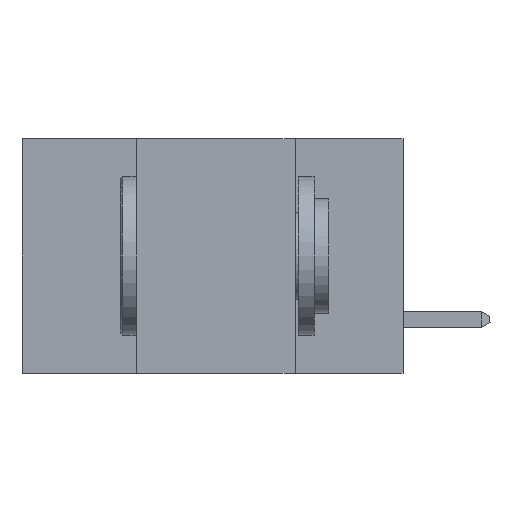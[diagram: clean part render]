
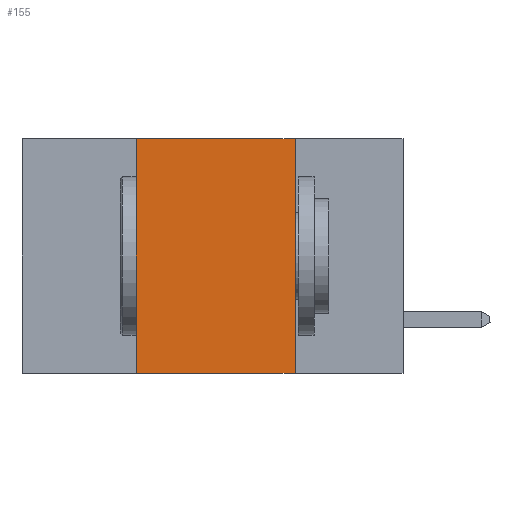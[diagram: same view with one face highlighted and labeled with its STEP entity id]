
A CAD part, left-side view. The second image highlights one B-rep face of the part: STEP entity #155.
In plain terms, the highlighted planar face has unit normal (-1, 0, 0).
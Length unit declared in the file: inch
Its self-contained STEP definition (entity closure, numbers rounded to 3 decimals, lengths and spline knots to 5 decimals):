
#155 = ADVANCED_FACE ( 'NONE', ( #1141 ), #7700, .F. ) ;
#547 = VERTEX_POINT ( 'NONE', #8016 ) ;
#861 = CARTESIAN_POINT ( 'NONE',  ( 0., 0.42, 0. ) ) ;
#939 = DIRECTION ( 'NONE',  ( 0., 0., -1. ) ) ;
#1141 = FACE_OUTER_BOUND ( 'NONE', #3780, .T. ) ;
#1144 = ORIENTED_EDGE ( 'NONE', *, *, #3062, .F. ) ;
#1249 = AXIS2_PLACEMENT_3D ( 'NONE', #10570, #8651, #9579 ) ;
#1253 = DIRECTION ( 'NONE',  ( 0., 0., 1. ) ) ;
#1817 = VERTEX_POINT ( 'NONE', #10960 ) ;
#2206 = EDGE_CURVE ( 'NONE', #1817, #547, #7486, .T. ) ;
#2218 = VECTOR ( 'NONE', #1253, 39.37008 ) ;
#2542 = VECTOR ( 'NONE', #939, 39.37008 ) ;
#3062 = EDGE_CURVE ( 'NONE', #9402, #5827, #3836, .T. ) ;
#3548 = EDGE_CURVE ( 'NONE', #5827, #1817, #9509, .T. ) ;
#3780 = EDGE_LOOP ( 'NONE', ( #6567, #8626, #1144, #9054 ) ) ;
#3836 = LINE ( 'NONE', #10677, #2218 ) ;
#4989 = EDGE_CURVE ( 'NONE', #9402, #547, #8886, .T. ) ;
#5162 = CARTESIAN_POINT ( 'NONE',  ( 0., 0.6, 0. ) ) ;
#5827 = VERTEX_POINT ( 'NONE', #861 ) ;
#5894 = DIRECTION ( 'NONE',  ( 0., -1., 0. ) ) ;
#6567 = ORIENTED_EDGE ( 'NONE', *, *, #2206, .F. ) ;
#7486 = LINE ( 'NONE', #8471, #2542 ) ;
#7700 = PLANE ( 'NONE',  #1249 ) ;
#8016 = CARTESIAN_POINT ( 'NONE',  ( 0., 0.17, -0.37 ) ) ;
#8092 = DIRECTION ( 'NONE',  ( 0., -1., 0. ) ) ;
#8471 = CARTESIAN_POINT ( 'NONE',  ( 0., 0.17, 0. ) ) ;
#8602 = VECTOR ( 'NONE', #5894, 39.37008 ) ;
#8626 = ORIENTED_EDGE ( 'NONE', *, *, #3548, .F. ) ;
#8651 = DIRECTION ( 'NONE',  ( 1., 0., 0. ) ) ;
#8886 = LINE ( 'NONE', #10516, #8602 ) ;
#9054 = ORIENTED_EDGE ( 'NONE', *, *, #4989, .T. ) ;
#9217 = VECTOR ( 'NONE', #8092, 39.37008 ) ;
#9402 = VERTEX_POINT ( 'NONE', #11376 ) ;
#9509 = LINE ( 'NONE', #5162, #9217 ) ;
#9579 = DIRECTION ( 'NONE',  ( 0., 0., -1. ) ) ;
#10516 = CARTESIAN_POINT ( 'NONE',  ( 0., 0.6, -0.37 ) ) ;
#10570 = CARTESIAN_POINT ( 'NONE',  ( 0., 0.6, 0. ) ) ;
#10677 = CARTESIAN_POINT ( 'NONE',  ( 0., 0.42, 0. ) ) ;
#10960 = CARTESIAN_POINT ( 'NONE',  ( 0., 0.17, 0. ) ) ;
#11376 = CARTESIAN_POINT ( 'NONE',  ( 0., 0.42, -0.37 ) ) ;
